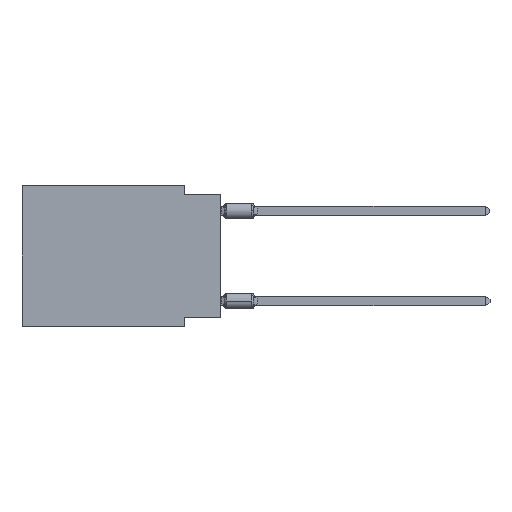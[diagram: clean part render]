
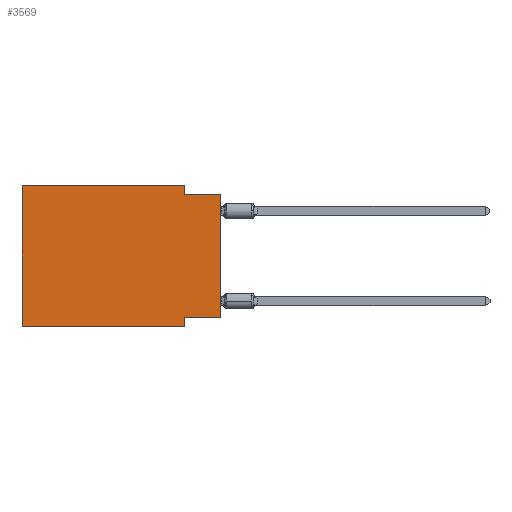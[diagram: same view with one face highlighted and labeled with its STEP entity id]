
A CAD part, left-side view. The second image highlights one B-rep face of the part: STEP entity #3569.
In plain terms, the highlighted planar face has unit normal (-1, 0, 0).
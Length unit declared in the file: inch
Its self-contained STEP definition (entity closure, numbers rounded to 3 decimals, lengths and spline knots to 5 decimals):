
#36 = AXIS2_PLACEMENT_3D ( 'NONE', #41269, #7225, #45402 ) ;
#1482 = ORIENTED_EDGE ( 'NONE', *, *, #8617, .T. ) ;
#2198 = LINE ( 'NONE', #47854, #5482 ) ;
#2731 = LINE ( 'NONE', #43118, #7170 ) ;
#2749 = LINE ( 'NONE', #25561, #40388 ) ;
#3123 = CARTESIAN_POINT ( 'NONE',  ( 0., 0.1, -0.025 ) ) ;
#3569 = ADVANCED_FACE ( 'NONE', ( #31932 ), #51719, .F. ) ;
#3799 = VECTOR ( 'NONE', #25358, 39.37008 ) ;
#3915 = VERTEX_POINT ( 'NONE', #40002 ) ;
#5421 = CARTESIAN_POINT ( 'NONE',  ( 0., 0.1, -0.39 ) ) ;
#5482 = VECTOR ( 'NONE', #16801, 39.37008 ) ;
#5551 = VERTEX_POINT ( 'NONE', #49580 ) ;
#7170 = VECTOR ( 'NONE', #57158, 39.37008 ) ;
#7225 = DIRECTION ( 'NONE',  ( 1., 0., 0. ) ) ;
#8617 = EDGE_CURVE ( 'NONE', #32635, #3915, #37451, .T. ) ;
#11712 = EDGE_CURVE ( 'NONE', #41661, #3915, #2198, .T. ) ;
#11818 = VERTEX_POINT ( 'NONE', #17670 ) ;
#12480 = LINE ( 'NONE', #20658, #57178 ) ;
#13465 = CARTESIAN_POINT ( 'NONE',  ( 0., 0.55, -0.39 ) ) ;
#14103 = VECTOR ( 'NONE', #23397, 39.37008 ) ;
#14619 = LINE ( 'NONE', #29250, #14103 ) ;
#16111 = ORIENTED_EDGE ( 'NONE', *, *, #17056, .T. ) ;
#16801 = DIRECTION ( 'NONE',  ( 0., -1., 0. ) ) ;
#17056 = EDGE_CURVE ( 'NONE', #39751, #41933, #40151, .T. ) ;
#17670 = CARTESIAN_POINT ( 'NONE',  ( 0., 0.1, 0. ) ) ;
#18638 = EDGE_LOOP ( 'NONE', ( #1482, #52225, #35338, #37494, #39964, #16111, #25720, #32799 ) ) ;
#19790 = VERTEX_POINT ( 'NONE', #51656 ) ;
#20658 = CARTESIAN_POINT ( 'NONE',  ( 0., 0.55, 0. ) ) ;
#22592 = VECTOR ( 'NONE', #40431, 39.37008 ) ;
#23397 = DIRECTION ( 'NONE',  ( 0., 1., 0. ) ) ;
#24248 = CARTESIAN_POINT ( 'NONE',  ( 0., 0., 0. ) ) ;
#25358 = DIRECTION ( 'NONE',  ( 0., 0., -1. ) ) ;
#25561 = CARTESIAN_POINT ( 'NONE',  ( 0., 0.1, -0.39 ) ) ;
#25720 = ORIENTED_EDGE ( 'NONE', *, *, #42067, .F. ) ;
#26273 = EDGE_CURVE ( 'NONE', #11818, #41661, #52892, .T. ) ;
#29250 = CARTESIAN_POINT ( 'NONE',  ( 0., 0., -0.365 ) ) ;
#29690 = DIRECTION ( 'NONE',  ( 0., 0., -1. ) ) ;
#31666 = CARTESIAN_POINT ( 'NONE',  ( 0., 0.55, -0.39 ) ) ;
#31932 = FACE_OUTER_BOUND ( 'NONE', #18638, .T. ) ;
#32635 = VERTEX_POINT ( 'NONE', #49772 ) ;
#32799 = ORIENTED_EDGE ( 'NONE', *, *, #41059, .F. ) ;
#35338 = ORIENTED_EDGE ( 'NONE', *, *, #26273, .F. ) ;
#37451 = LINE ( 'NONE', #24248, #55752 ) ;
#37494 = ORIENTED_EDGE ( 'NONE', *, *, #41589, .F. ) ;
#38851 = CARTESIAN_POINT ( 'NONE',  ( 0., 0.1, 0. ) ) ;
#39751 = VERTEX_POINT ( 'NONE', #13465 ) ;
#39964 = ORIENTED_EDGE ( 'NONE', *, *, #49962, .F. ) ;
#40002 = CARTESIAN_POINT ( 'NONE',  ( 0., 0., -0.025 ) ) ;
#40151 = LINE ( 'NONE', #31666, #22592 ) ;
#40388 = VECTOR ( 'NONE', #29690, 39.37008 ) ;
#40431 = DIRECTION ( 'NONE',  ( 0., -1., 0. ) ) ;
#41059 = EDGE_CURVE ( 'NONE', #32635, #19790, #14619, .T. ) ;
#41269 = CARTESIAN_POINT ( 'NONE',  ( 0., 0.55, 0. ) ) ;
#41589 = EDGE_CURVE ( 'NONE', #5551, #11818, #12480, .T. ) ;
#41661 = VERTEX_POINT ( 'NONE', #3123 ) ;
#41933 = VERTEX_POINT ( 'NONE', #5421 ) ;
#42067 = EDGE_CURVE ( 'NONE', #19790, #41933, #2749, .T. ) ;
#43118 = CARTESIAN_POINT ( 'NONE',  ( 0., 0.55, 0. ) ) ;
#45402 = DIRECTION ( 'NONE',  ( 0., 0., -1. ) ) ;
#46815 = DIRECTION ( 'NONE',  ( 0., 0., 1. ) ) ;
#47854 = CARTESIAN_POINT ( 'NONE',  ( 0., 0., -0.025 ) ) ;
#49580 = CARTESIAN_POINT ( 'NONE',  ( 0., 0.55, 0. ) ) ;
#49772 = CARTESIAN_POINT ( 'NONE',  ( 0., 0., -0.365 ) ) ;
#49962 = EDGE_CURVE ( 'NONE', #39751, #5551, #2731, .T. ) ;
#51656 = CARTESIAN_POINT ( 'NONE',  ( 0., 0.1, -0.365 ) ) ;
#51719 = PLANE ( 'NONE',  #36 ) ;
#52225 = ORIENTED_EDGE ( 'NONE', *, *, #11712, .F. ) ;
#52892 = LINE ( 'NONE', #38851, #3799 ) ;
#55752 = VECTOR ( 'NONE', #46815, 39.37008 ) ;
#56381 = DIRECTION ( 'NONE',  ( 0., -1., 0. ) ) ;
#57158 = DIRECTION ( 'NONE',  ( 0., 0., 1. ) ) ;
#57178 = VECTOR ( 'NONE', #56381, 39.37008 ) ;
